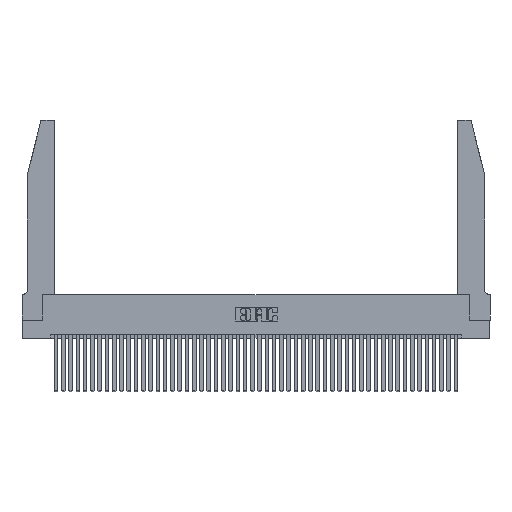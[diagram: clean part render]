
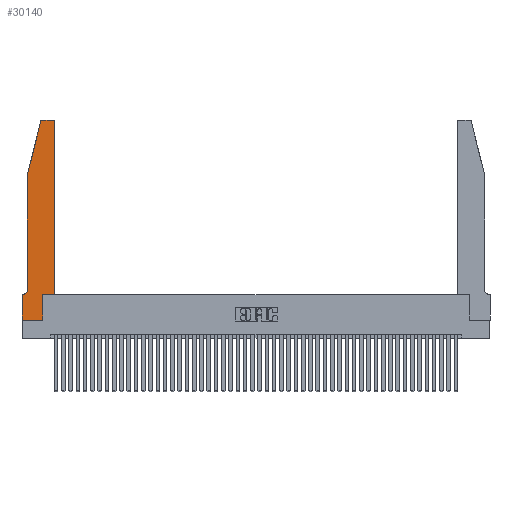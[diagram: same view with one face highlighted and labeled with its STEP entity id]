
A CAD part, top view. The second image highlights one B-rep face of the part: STEP entity #30140.
In plain terms, the highlighted planar face has unit normal (0, 0, 1).
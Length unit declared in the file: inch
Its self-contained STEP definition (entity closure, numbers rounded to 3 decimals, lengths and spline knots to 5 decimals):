
#812 = EDGE_CURVE ( 'NONE', #36094, #17669, #11748, .T. ) ;
#1741 = VECTOR ( 'NONE', #13616, 39.37008 ) ;
#2513 = CARTESIAN_POINT ( 'NONE',  ( 0., 0., 0.37 ) ) ;
#3627 = DIRECTION ( 'NONE',  ( 0., 0., 1. ) ) ;
#4080 = CARTESIAN_POINT ( 'NONE',  ( 0.0755, 0.42, 0.37 ) ) ;
#4196 = CARTESIAN_POINT ( 'NONE',  ( 0.4505, 2.72, 0.37 ) ) ;
#4382 = LINE ( 'NONE', #37912, #32099 ) ;
#7006 = ORIENTED_EDGE ( 'NONE', *, *, #44344, .T. ) ;
#7211 = CARTESIAN_POINT ( 'NONE',  ( 0.0755, 0.35, 0.37 ) ) ;
#7334 = CARTESIAN_POINT ( 'NONE',  ( 0., 0.35, 0.37 ) ) ;
#7417 = VECTOR ( 'NONE', #43122, 39.37008 ) ;
#7517 = DIRECTION ( 'NONE',  ( -0.239, -0.971, 0. ) ) ;
#7594 = ORIENTED_EDGE ( 'NONE', *, *, #36371, .T. ) ;
#7799 = VERTEX_POINT ( 'NONE', #14211 ) ;
#8435 = CIRCLE ( 'NONE', #36939, 0.03 ) ;
#10678 = DIRECTION ( 'NONE',  ( 0., 1., 0. ) ) ;
#10927 = CARTESIAN_POINT ( 'NONE',  ( 0.4205, 2.72, 0.37 ) ) ;
#11014 = DIRECTION ( 'NONE',  ( 1., 0., 0. ) ) ;
#11019 = EDGE_CURVE ( 'NONE', #7799, #36677, #40675, .T. ) ;
#11188 = CARTESIAN_POINT ( 'NONE',  ( 0.0755, 2., 0.37 ) ) ;
#11486 = LINE ( 'NONE', #2513, #1741 ) ;
#11549 = VECTOR ( 'NONE', #10678, 39.37008 ) ;
#11709 = CARTESIAN_POINT ( 'NONE',  ( 0.0055, 0.42, 0.37 ) ) ;
#11748 = LINE ( 'NONE', #41724, #29759 ) ;
#12528 = DIRECTION ( 'NONE',  ( -1., 0., 0. ) ) ;
#13338 = ORIENTED_EDGE ( 'NONE', *, *, #35009, .T. ) ;
#13616 = DIRECTION ( 'NONE',  ( 1., 0., 0. ) ) ;
#13822 = EDGE_CURVE ( 'NONE', #17782, #36094, #4382, .T. ) ;
#14211 = CARTESIAN_POINT ( 'NONE',  ( 0.25487, 2.72718, 0.37 ) ) ;
#14677 = DIRECTION ( 'NONE',  ( 1., 0., 0. ) ) ;
#14724 = EDGE_CURVE ( 'NONE', #42380, #17782, #29581, .T. ) ;
#14777 = EDGE_CURVE ( 'NONE', #30748, #7799, #39010, .T. ) ;
#15020 = VERTEX_POINT ( 'NONE', #19275 ) ;
#15421 = DIRECTION ( 'NONE',  ( -1., 0., 0. ) ) ;
#16163 = ORIENTED_EDGE ( 'NONE', *, *, #23088, .T. ) ;
#16558 = DIRECTION ( 'NONE',  ( 1., 0., 0. ) ) ;
#17157 = LINE ( 'NONE', #7211, #7417 ) ;
#17669 = VERTEX_POINT ( 'NONE', #4196 ) ;
#17782 = VERTEX_POINT ( 'NONE', #44414 ) ;
#18914 = CARTESIAN_POINT ( 'NONE',  ( 0.0755, 2., 0.37 ) ) ;
#18967 = VERTEX_POINT ( 'NONE', #4080 ) ;
#18972 = CARTESIAN_POINT ( 'NONE',  ( 0., 0., 0.37 ) ) ;
#19275 = CARTESIAN_POINT ( 'NONE',  ( 0., 0.35, 0.37 ) ) ;
#19541 = ORIENTED_EDGE ( 'NONE', *, *, #33325, .T. ) ;
#22545 = DIRECTION ( 'NONE',  ( 0., -1., 0. ) ) ;
#23088 = EDGE_CURVE ( 'NONE', #36677, #18967, #39474, .T. ) ;
#23411 = CARTESIAN_POINT ( 'NONE',  ( 0.2605, 2.75, 0.37 ) ) ;
#25377 = CARTESIAN_POINT ( 'NONE',  ( 0.284, 2.72, 0.37 ) ) ;
#25723 = ORIENTED_EDGE ( 'NONE', *, *, #812, .T. ) ;
#26008 = DIRECTION ( 'NONE',  ( 0., -1., 0. ) ) ;
#26174 = VECTOR ( 'NONE', #12528, 39.37008 ) ;
#26753 = PLANE ( 'NONE',  #33827 ) ;
#26980 = FACE_OUTER_BOUND ( 'NONE', #35827, .T. ) ;
#28507 = ORIENTED_EDGE ( 'NONE', *, *, #14724, .T. ) ;
#28982 = DIRECTION ( 'NONE',  ( 1., 0., 0. ) ) ;
#29581 = LINE ( 'NONE', #32256, #11549 ) ;
#29759 = VECTOR ( 'NONE', #38175, 39.37008 ) ;
#30059 = VECTOR ( 'NONE', #22545, 39.37008 ) ;
#30132 = VECTOR ( 'NONE', #7517, 39.37008 ) ;
#30140 = ADVANCED_FACE ( 'NONE', ( #26980 ), #26753, .T. ) ;
#30720 = ORIENTED_EDGE ( 'NONE', *, *, #11019, .T. ) ;
#30748 = VERTEX_POINT ( 'NONE', #42433 ) ;
#30785 = CARTESIAN_POINT ( 'NONE',  ( 0.4205, 2.75, 0.37 ) ) ;
#31820 = VECTOR ( 'NONE', #26008, 39.37008 ) ;
#31871 = ORIENTED_EDGE ( 'NONE', *, *, #13822, .T. ) ;
#32043 = EDGE_CURVE ( 'NONE', #15020, #40091, #34040, .T. ) ;
#32099 = VECTOR ( 'NONE', #16558, 39.37008 ) ;
#32256 = CARTESIAN_POINT ( 'NONE',  ( 0.2865, 0.35, 0.37 ) ) ;
#32390 = ORIENTED_EDGE ( 'NONE', *, *, #32043, .T. ) ;
#32562 = DIRECTION ( 'NONE',  ( 0., 0., 1. ) ) ;
#32997 = AXIS2_PLACEMENT_3D ( 'NONE', #11709, #36787, #15421 ) ;
#33183 = CARTESIAN_POINT ( 'NONE',  ( 0.2865, 0., 0.37 ) ) ;
#33325 = EDGE_CURVE ( 'NONE', #18967, #44610, #45102, .T. ) ;
#33369 = EDGE_CURVE ( 'NONE', #34709, #30748, #41729, .T. ) ;
#33827 = AXIS2_PLACEMENT_3D ( 'NONE', #7334, #32562, #11014 ) ;
#34040 = LINE ( 'NONE', #18972, #31820 ) ;
#34539 = CARTESIAN_POINT ( 'NONE',  ( 0.4505, 0.35, 0.37 ) ) ;
#34709 = VERTEX_POINT ( 'NONE', #30785 ) ;
#35009 = EDGE_CURVE ( 'NONE', #44610, #15020, #17157, .T. ) ;
#35827 = EDGE_LOOP ( 'NONE', ( #36783, #46247, #30720, #16163, #19541, #13338, #32390, #7006, #28507, #31871, #25723, #7594 ) ) ;
#36039 = DIRECTION ( 'NONE',  ( 0., 0., 1. ) ) ;
#36094 = VERTEX_POINT ( 'NONE', #34539 ) ;
#36371 = EDGE_CURVE ( 'NONE', #17669, #34709, #8435, .T. ) ;
#36677 = VERTEX_POINT ( 'NONE', #44568 ) ;
#36783 = ORIENTED_EDGE ( 'NONE', *, *, #33369, .T. ) ;
#36787 = DIRECTION ( 'NONE',  ( 0., 0., -1. ) ) ;
#36939 = AXIS2_PLACEMENT_3D ( 'NONE', #10927, #36039, #14677 ) ;
#37912 = CARTESIAN_POINT ( 'NONE',  ( 0.4505, 0.35, 0.37 ) ) ;
#38175 = DIRECTION ( 'NONE',  ( 0., 1., 0. ) ) ;
#39010 = CIRCLE ( 'NONE', #46106, 0.03 ) ;
#39474 = LINE ( 'NONE', #18914, #30059 ) ;
#40091 = VERTEX_POINT ( 'NONE', #46358 ) ;
#40675 = LINE ( 'NONE', #11188, #30132 ) ;
#41724 = CARTESIAN_POINT ( 'NONE',  ( 0.4505, 0.35, 0.37 ) ) ;
#41729 = LINE ( 'NONE', #23411, #26174 ) ;
#42380 = VERTEX_POINT ( 'NONE', #33183 ) ;
#42433 = CARTESIAN_POINT ( 'NONE',  ( 0.284, 2.75, 0.37 ) ) ;
#43122 = DIRECTION ( 'NONE',  ( -1., 0., 0. ) ) ;
#43364 = CARTESIAN_POINT ( 'NONE',  ( 0.0055, 0.35, 0.37 ) ) ;
#44344 = EDGE_CURVE ( 'NONE', #40091, #42380, #11486, .T. ) ;
#44414 = CARTESIAN_POINT ( 'NONE',  ( 0.2865, 0.35, 0.37 ) ) ;
#44568 = CARTESIAN_POINT ( 'NONE',  ( 0.0755, 2., 0.37 ) ) ;
#44610 = VERTEX_POINT ( 'NONE', #43364 ) ;
#45102 = CIRCLE ( 'NONE', #32997, 0.07 ) ;
#46106 = AXIS2_PLACEMENT_3D ( 'NONE', #25377, #3627, #28982 ) ;
#46247 = ORIENTED_EDGE ( 'NONE', *, *, #14777, .T. ) ;
#46358 = CARTESIAN_POINT ( 'NONE',  ( 0., 0., 0.37 ) ) ;
